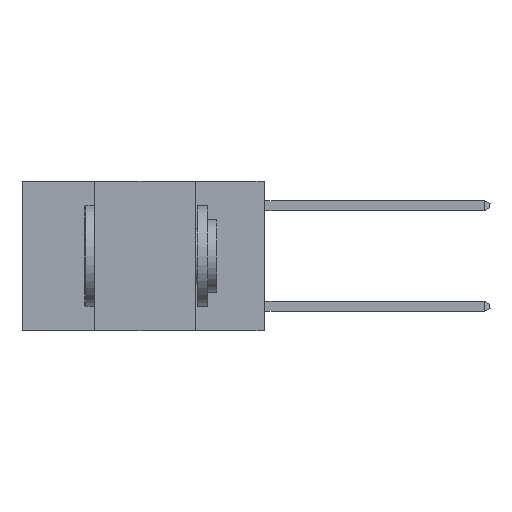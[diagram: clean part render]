
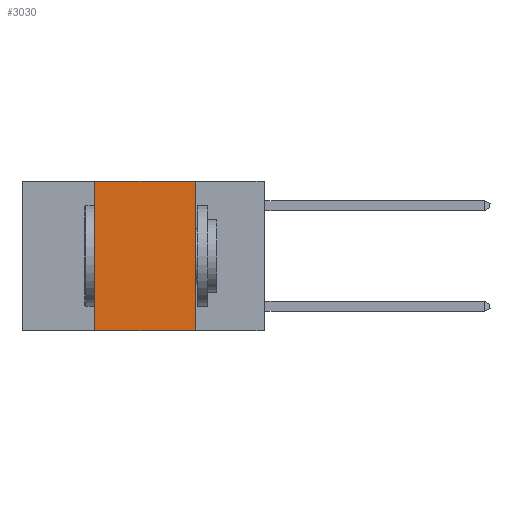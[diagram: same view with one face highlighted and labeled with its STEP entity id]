
A CAD part, left-side view. The second image highlights one B-rep face of the part: STEP entity #3030.
In plain terms, the highlighted planar face has unit normal (-1, 0, 0).
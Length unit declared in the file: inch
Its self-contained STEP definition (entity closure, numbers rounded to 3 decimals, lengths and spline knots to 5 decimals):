
#325 = CARTESIAN_POINT ( 'NONE',  ( 0., 0.6, 0. ) ) ;
#1883 = CARTESIAN_POINT ( 'NONE',  ( 0., 0.42, 0. ) ) ;
#2351 = LINE ( 'NONE', #12875, #13793 ) ;
#3030 = ADVANCED_FACE ( 'NONE', ( #17512 ), #11063, .F. ) ;
#4948 = LINE ( 'NONE', #6410, #6026 ) ;
#6026 = VECTOR ( 'NONE', #9313, 39.37008 ) ;
#6410 = CARTESIAN_POINT ( 'NONE',  ( 0., 0.6, 0. ) ) ;
#6602 = EDGE_CURVE ( 'NONE', #7501, #7870, #10261, .T. ) ;
#6619 = DIRECTION ( 'NONE',  ( 0., 0., -1. ) ) ;
#7206 = EDGE_LOOP ( 'NONE', ( #19144, #16452, #14611, #20024 ) ) ;
#7228 = EDGE_CURVE ( 'NONE', #7501, #17735, #8977, .T. ) ;
#7501 = VERTEX_POINT ( 'NONE', #13557 ) ;
#7730 = CARTESIAN_POINT ( 'NONE',  ( 0., 0.17, 0. ) ) ;
#7870 = VERTEX_POINT ( 'NONE', #1883 ) ;
#7951 = DIRECTION ( 'NONE',  ( 1., 0., 0. ) ) ;
#8546 = DIRECTION ( 'NONE',  ( 0., 0., -1. ) ) ;
#8590 = CARTESIAN_POINT ( 'NONE',  ( 0., 0.42, 0. ) ) ;
#8969 = VERTEX_POINT ( 'NONE', #7730 ) ;
#8977 = LINE ( 'NONE', #10947, #13146 ) ;
#9313 = DIRECTION ( 'NONE',  ( 0., -1., 0. ) ) ;
#9646 = CARTESIAN_POINT ( 'NONE',  ( 0., 0.17, -0.37 ) ) ;
#10261 = LINE ( 'NONE', #8590, #12128 ) ;
#10947 = CARTESIAN_POINT ( 'NONE',  ( 0., 0.6, -0.37 ) ) ;
#11063 = PLANE ( 'NONE',  #16836 ) ;
#12066 = DIRECTION ( 'NONE',  ( 0., -1., 0. ) ) ;
#12128 = VECTOR ( 'NONE', #14857, 39.37008 ) ;
#12266 = EDGE_CURVE ( 'NONE', #8969, #17735, #2351, .T. ) ;
#12875 = CARTESIAN_POINT ( 'NONE',  ( 0., 0.17, 0. ) ) ;
#13146 = VECTOR ( 'NONE', #12066, 39.37008 ) ;
#13557 = CARTESIAN_POINT ( 'NONE',  ( 0., 0.42, -0.37 ) ) ;
#13793 = VECTOR ( 'NONE', #8546, 39.37008 ) ;
#14611 = ORIENTED_EDGE ( 'NONE', *, *, #6602, .F. ) ;
#14857 = DIRECTION ( 'NONE',  ( 0., 0., 1. ) ) ;
#16452 = ORIENTED_EDGE ( 'NONE', *, *, #19371, .F. ) ;
#16836 = AXIS2_PLACEMENT_3D ( 'NONE', #325, #7951, #6619 ) ;
#17512 = FACE_OUTER_BOUND ( 'NONE', #7206, .T. ) ;
#17735 = VERTEX_POINT ( 'NONE', #9646 ) ;
#19144 = ORIENTED_EDGE ( 'NONE', *, *, #12266, .F. ) ;
#19371 = EDGE_CURVE ( 'NONE', #7870, #8969, #4948, .T. ) ;
#20024 = ORIENTED_EDGE ( 'NONE', *, *, #7228, .T. ) ;
